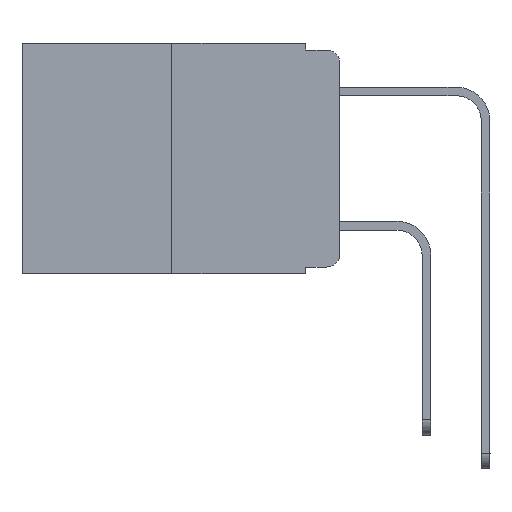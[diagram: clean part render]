
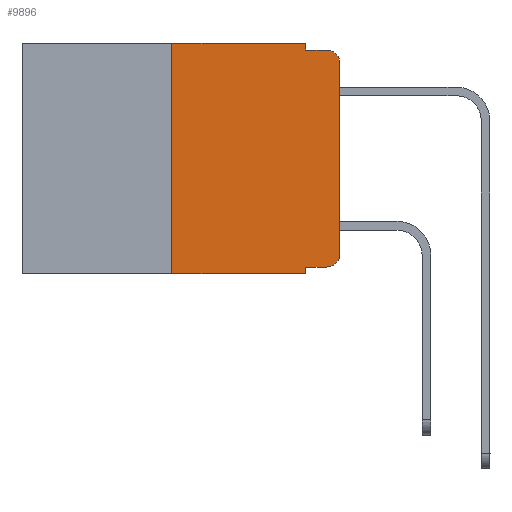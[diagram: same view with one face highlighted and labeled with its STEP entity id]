
A CAD part, left-side view. The second image highlights one B-rep face of the part: STEP entity #9896.
In plain terms, the highlighted planar face has unit normal (-1, 0, 0).
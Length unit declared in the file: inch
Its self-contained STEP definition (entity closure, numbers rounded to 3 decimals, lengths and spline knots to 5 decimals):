
#148 = VERTEX_POINT ( 'NONE', #6461 ) ;
#201 = DIRECTION ( 'NONE',  ( 0., 0., -1. ) ) ;
#580 = DIRECTION ( 'NONE',  ( 0., 0., -1. ) ) ;
#832 = DIRECTION ( 'NONE',  ( 0., 0., 1. ) ) ;
#903 = VERTEX_POINT ( 'NONE', #21155 ) ;
#935 = ORIENTED_EDGE ( 'NONE', *, *, #17987, .F. ) ;
#1754 = EDGE_CURVE ( 'NONE', #20887, #903, #16734, .T. ) ;
#1828 = CARTESIAN_POINT ( 'NONE',  ( 0., 0.25, 0. ) ) ;
#2137 = EDGE_CURVE ( 'NONE', #11962, #25694, #5364, .T. ) ;
#2232 = VECTOR ( 'NONE', #201, 39.37008 ) ;
#2314 = AXIS2_PLACEMENT_3D ( 'NONE', #24260, #9876, #20232 ) ;
#2413 = CARTESIAN_POINT ( 'NONE',  ( 0., 0.051, 0. ) ) ;
#2929 = ORIENTED_EDGE ( 'NONE', *, *, #24489, .F. ) ;
#3151 = DIRECTION ( 'NONE',  ( 0., -1., 0. ) ) ;
#3223 = CIRCLE ( 'NONE', #24857, 0.02 ) ;
#3713 = ORIENTED_EDGE ( 'NONE', *, *, #1754, .F. ) ;
#5364 = LINE ( 'NONE', #26650, #12165 ) ;
#5395 = ORIENTED_EDGE ( 'NONE', *, *, #9087, .T. ) ;
#6289 = LINE ( 'NONE', #2413, #2232 ) ;
#6461 = CARTESIAN_POINT ( 'NONE',  ( 0., 0., -0.03 ) ) ;
#7671 = VECTOR ( 'NONE', #25319, 39.37008 ) ;
#8150 = CARTESIAN_POINT ( 'NONE',  ( 0., 0.051, -0.343 ) ) ;
#8510 = CARTESIAN_POINT ( 'NONE',  ( 0., 0.25, -0.343 ) ) ;
#9087 = EDGE_CURVE ( 'NONE', #26407, #27103, #14551, .T. ) ;
#9876 = DIRECTION ( 'NONE',  ( 1., 0., 0. ) ) ;
#9894 = EDGE_CURVE ( 'NONE', #27103, #26387, #19158, .T. ) ;
#9896 = ADVANCED_FACE ( 'NONE', ( #22306 ), #13599, .F. ) ;
#10870 = VERTEX_POINT ( 'NONE', #8510 ) ;
#11551 = VECTOR ( 'NONE', #24868, 39.37008 ) ;
#11881 = VECTOR ( 'NONE', #832, 39.37008 ) ;
#11921 = CARTESIAN_POINT ( 'NONE',  ( 0., 0.051, 0. ) ) ;
#11962 = VERTEX_POINT ( 'NONE', #24167 ) ;
#12073 = CARTESIAN_POINT ( 'NONE',  ( 0., 0.051, -0.333 ) ) ;
#12165 = VECTOR ( 'NONE', #3151, 39.37008 ) ;
#12203 = LINE ( 'NONE', #1828, #13555 ) ;
#13269 = ORIENTED_EDGE ( 'NONE', *, *, #20630, .T. ) ;
#13555 = VECTOR ( 'NONE', #14129, 39.37008 ) ;
#13599 = PLANE ( 'NONE',  #2314 ) ;
#13633 = CARTESIAN_POINT ( 'NONE',  ( 0., 0.051, -0.01 ) ) ;
#13730 = LINE ( 'NONE', #11921, #25289 ) ;
#13782 = EDGE_LOOP ( 'NONE', ( #21127, #25841, #3713, #935, #22022, #17614, #13269, #2929, #5395, #20077 ) ) ;
#14081 = EDGE_CURVE ( 'NONE', #10870, #11962, #12203, .T. ) ;
#14129 = DIRECTION ( 'NONE',  ( 0., 0., 1. ) ) ;
#14551 = LINE ( 'NONE', #12073, #24021 ) ;
#15817 = DIRECTION ( 'NONE',  ( 0., 0., -1. ) ) ;
#16283 = EDGE_CURVE ( 'NONE', #26387, #148, #19779, .T. ) ;
#16734 = LINE ( 'NONE', #16868, #7671 ) ;
#16868 = CARTESIAN_POINT ( 'NONE',  ( 0., 0.051, -0.01 ) ) ;
#17305 = CARTESIAN_POINT ( 'NONE',  ( 0., 0.02, -0.03 ) ) ;
#17614 = ORIENTED_EDGE ( 'NONE', *, *, #14081, .F. ) ;
#17987 = EDGE_CURVE ( 'NONE', #25694, #20887, #6289, .T. ) ;
#18805 = CARTESIAN_POINT ( 'NONE',  ( 0., 0., -0.313 ) ) ;
#19158 = CIRCLE ( 'NONE', #23127, 0.02 ) ;
#19515 = DIRECTION ( 'NONE',  ( -1., 0., 0. ) ) ;
#19779 = LINE ( 'NONE', #26428, #11881 ) ;
#20077 = ORIENTED_EDGE ( 'NONE', *, *, #9894, .T. ) ;
#20232 = DIRECTION ( 'NONE',  ( 0., 0., -1. ) ) ;
#20630 = EDGE_CURVE ( 'NONE', #10870, #25615, #21113, .T. ) ;
#20645 = DIRECTION ( 'NONE',  ( 0., 0., -1. ) ) ;
#20887 = VERTEX_POINT ( 'NONE', #13633 ) ;
#21064 = DIRECTION ( 'NONE',  ( 0., -1., 0. ) ) ;
#21113 = LINE ( 'NONE', #25274, #11551 ) ;
#21127 = ORIENTED_EDGE ( 'NONE', *, *, #16283, .T. ) ;
#21155 = CARTESIAN_POINT ( 'NONE',  ( 0., 0.02, -0.01 ) ) ;
#21395 = CARTESIAN_POINT ( 'NONE',  ( 0., 0.051, 0. ) ) ;
#22022 = ORIENTED_EDGE ( 'NONE', *, *, #2137, .F. ) ;
#22306 = FACE_OUTER_BOUND ( 'NONE', #13782, .T. ) ;
#22727 = CARTESIAN_POINT ( 'NONE',  ( 0., 0.02, -0.333 ) ) ;
#23083 = CARTESIAN_POINT ( 'NONE',  ( 0., 0.051, -0.333 ) ) ;
#23127 = AXIS2_PLACEMENT_3D ( 'NONE', #25038, #24386, #15817 ) ;
#24021 = VECTOR ( 'NONE', #21064, 39.37008 ) ;
#24167 = CARTESIAN_POINT ( 'NONE',  ( 0., 0.25, 0. ) ) ;
#24260 = CARTESIAN_POINT ( 'NONE',  ( 0., 0.473, 0. ) ) ;
#24386 = DIRECTION ( 'NONE',  ( -1., 0., 0. ) ) ;
#24489 = EDGE_CURVE ( 'NONE', #26407, #25615, #13730, .T. ) ;
#24828 = EDGE_CURVE ( 'NONE', #148, #903, #3223, .T. ) ;
#24857 = AXIS2_PLACEMENT_3D ( 'NONE', #17305, #19515, #580 ) ;
#24868 = DIRECTION ( 'NONE',  ( 0., -1., 0. ) ) ;
#25038 = CARTESIAN_POINT ( 'NONE',  ( 0., 0.02, -0.313 ) ) ;
#25274 = CARTESIAN_POINT ( 'NONE',  ( 0., 0.473, -0.343 ) ) ;
#25289 = VECTOR ( 'NONE', #20645, 39.37008 ) ;
#25319 = DIRECTION ( 'NONE',  ( 0., -1., 0. ) ) ;
#25615 = VERTEX_POINT ( 'NONE', #8150 ) ;
#25694 = VERTEX_POINT ( 'NONE', #21395 ) ;
#25841 = ORIENTED_EDGE ( 'NONE', *, *, #24828, .T. ) ;
#26387 = VERTEX_POINT ( 'NONE', #18805 ) ;
#26407 = VERTEX_POINT ( 'NONE', #23083 ) ;
#26428 = CARTESIAN_POINT ( 'NONE',  ( 0., 0., 0. ) ) ;
#26650 = CARTESIAN_POINT ( 'NONE',  ( 0., 0.473, 0. ) ) ;
#27103 = VERTEX_POINT ( 'NONE', #22727 ) ;
